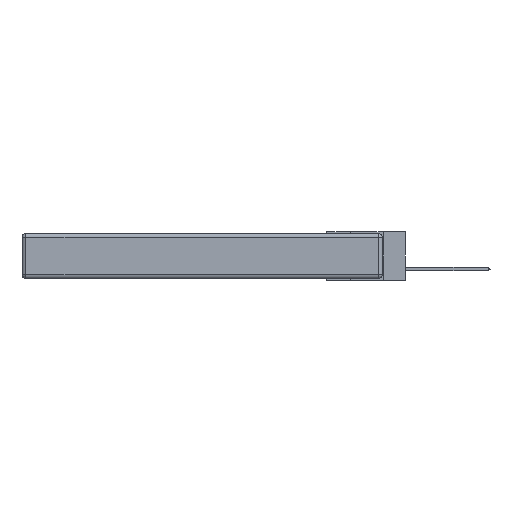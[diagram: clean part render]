
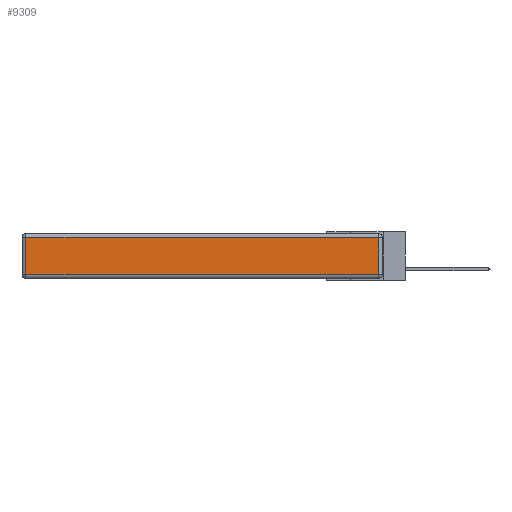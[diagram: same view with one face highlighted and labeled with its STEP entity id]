
A CAD part, left-side view. The second image highlights one B-rep face of the part: STEP entity #9309.
In plain terms, the highlighted planar face has unit normal (-1, 0, 0).
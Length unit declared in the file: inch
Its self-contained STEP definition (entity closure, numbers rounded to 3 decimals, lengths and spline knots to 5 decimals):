
#94 = ORIENTED_EDGE ( 'NONE', *, *, #1140, .T. ) ;
#486 = CARTESIAN_POINT ( 'NONE',  ( 0., 2.72, -0.313 ) ) ;
#1140 = EDGE_CURVE ( 'NONE', #19395, #8677, #17129, .T. ) ;
#1584 = CARTESIAN_POINT ( 'NONE',  ( 0., 2.75, -0.03 ) ) ;
#3255 = CARTESIAN_POINT ( 'NONE',  ( 0., 0.03, -0.03 ) ) ;
#4058 = ORIENTED_EDGE ( 'NONE', *, *, #10896, .T. ) ;
#4507 = DIRECTION ( 'NONE',  ( 0., 0., 1. ) ) ;
#5769 = AXIS2_PLACEMENT_3D ( 'NONE', #12573, #20183, #10587 ) ;
#7932 = EDGE_CURVE ( 'NONE', #8677, #16464, #23514, .T. ) ;
#8677 = VERTEX_POINT ( 'NONE', #486 ) ;
#9309 = ADVANCED_FACE ( 'NONE', ( #12527 ), #12255, .T. ) ;
#9332 = EDGE_CURVE ( 'NONE', #13601, #19395, #15177, .T. ) ;
#9904 = CARTESIAN_POINT ( 'NONE',  ( 0., 0.03, -0.343 ) ) ;
#10154 = VECTOR ( 'NONE', #20344, 39.37008 ) ;
#10587 = DIRECTION ( 'NONE',  ( 0., 0., 1. ) ) ;
#10896 = EDGE_CURVE ( 'NONE', #16464, #13601, #16289, .T. ) ;
#10959 = EDGE_LOOP ( 'NONE', ( #11135, #4058, #15158, #94 ) ) ;
#11135 = ORIENTED_EDGE ( 'NONE', *, *, #7932, .T. ) ;
#12255 = PLANE ( 'NONE',  #5769 ) ;
#12415 = CARTESIAN_POINT ( 'NONE',  ( 0., 0.03, -0.313 ) ) ;
#12527 = FACE_OUTER_BOUND ( 'NONE', #10959, .T. ) ;
#12573 = CARTESIAN_POINT ( 'NONE',  ( 0., 0., -0.343 ) ) ;
#13601 = VERTEX_POINT ( 'NONE', #3255 ) ;
#15158 = ORIENTED_EDGE ( 'NONE', *, *, #9332, .T. ) ;
#15177 = LINE ( 'NONE', #1584, #10154 ) ;
#16289 = LINE ( 'NONE', #9904, #24190 ) ;
#16464 = VERTEX_POINT ( 'NONE', #12415 ) ;
#17129 = LINE ( 'NONE', #22561, #21538 ) ;
#17824 = CARTESIAN_POINT ( 'NONE',  ( 0., 0., -0.313 ) ) ;
#18936 = DIRECTION ( 'NONE',  ( 0., 0., -1. ) ) ;
#19395 = VERTEX_POINT ( 'NONE', #22924 ) ;
#19565 = DIRECTION ( 'NONE',  ( 0., -1., 0. ) ) ;
#20183 = DIRECTION ( 'NONE',  ( -1., 0., 0. ) ) ;
#20344 = DIRECTION ( 'NONE',  ( 0., 1., 0. ) ) ;
#21538 = VECTOR ( 'NONE', #18936, 39.37008 ) ;
#22561 = CARTESIAN_POINT ( 'NONE',  ( 0., 2.72, -0.343 ) ) ;
#22924 = CARTESIAN_POINT ( 'NONE',  ( 0., 2.72, -0.03 ) ) ;
#22925 = VECTOR ( 'NONE', #19565, 39.37008 ) ;
#23514 = LINE ( 'NONE', #17824, #22925 ) ;
#24190 = VECTOR ( 'NONE', #4507, 39.37008 ) ;
